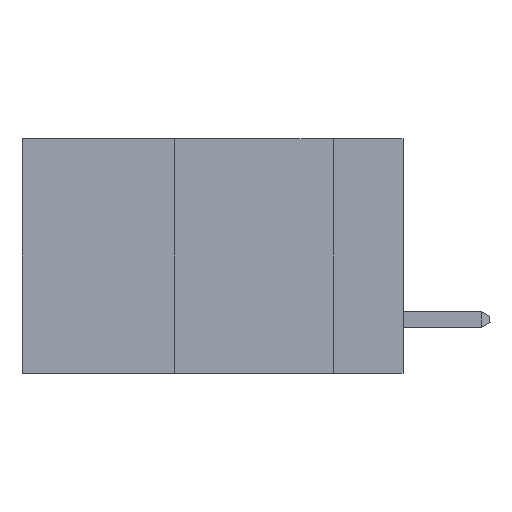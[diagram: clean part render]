
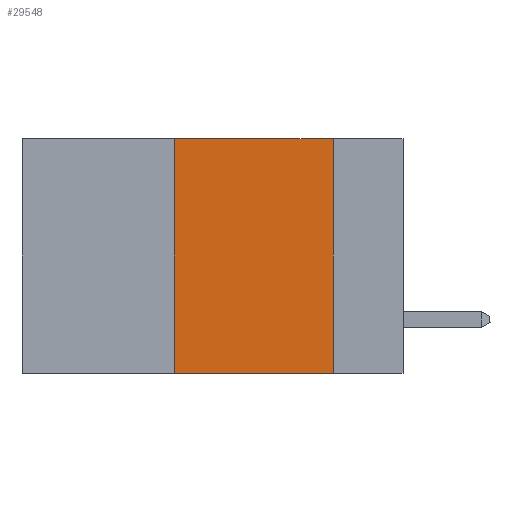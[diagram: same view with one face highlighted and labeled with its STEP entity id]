
A CAD part, left-side view. The second image highlights one B-rep face of the part: STEP entity #29548.
In plain terms, the highlighted planar face has unit normal (-1, 0, 0).
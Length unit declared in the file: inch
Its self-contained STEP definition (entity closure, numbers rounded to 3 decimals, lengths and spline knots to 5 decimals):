
#2512 = DIRECTION ( 'NONE',  ( 0., -1., 0. ) ) ;
#3248 = EDGE_CURVE ( 'NONE', #17567, #26143, #38191, .T. ) ;
#7248 = ORIENTED_EDGE ( 'NONE', *, *, #3248, .T. ) ;
#9143 = FACE_OUTER_BOUND ( 'NONE', #29233, .T. ) ;
#9183 = VECTOR ( 'NONE', #2512, 39.37008 ) ;
#13706 = VECTOR ( 'NONE', #22675, 39.37008 ) ;
#14139 = ORIENTED_EDGE ( 'NONE', *, *, #31482, .F. ) ;
#14521 = CARTESIAN_POINT ( 'NONE',  ( 0., 0.6, 0. ) ) ;
#14981 = LINE ( 'NONE', #34038, #13706 ) ;
#17039 = DIRECTION ( 'NONE',  ( 0., -1., 0. ) ) ;
#17567 = VERTEX_POINT ( 'NONE', #29278 ) ;
#18116 = LINE ( 'NONE', #24671, #36914 ) ;
#18705 = VERTEX_POINT ( 'NONE', #47653 ) ;
#19003 = LINE ( 'NONE', #14521, #9183 ) ;
#21620 = AXIS2_PLACEMENT_3D ( 'NONE', #41394, #22061, #49184 ) ;
#22061 = DIRECTION ( 'NONE',  ( 1., 0., 0. ) ) ;
#22595 = ORIENTED_EDGE ( 'NONE', *, *, #48093, .F. ) ;
#22675 = DIRECTION ( 'NONE',  ( 0., 0., 1. ) ) ;
#24671 = CARTESIAN_POINT ( 'NONE',  ( 0., 0.11, 0. ) ) ;
#26143 = VERTEX_POINT ( 'NONE', #26427 ) ;
#26427 = CARTESIAN_POINT ( 'NONE',  ( 0., 0.11, -0.37 ) ) ;
#27709 = DIRECTION ( 'NONE',  ( 0., 0., -1. ) ) ;
#29233 = EDGE_LOOP ( 'NONE', ( #14139, #22595, #47042, #7248 ) ) ;
#29278 = CARTESIAN_POINT ( 'NONE',  ( 0., 0.36, -0.37 ) ) ;
#29548 = ADVANCED_FACE ( 'NONE', ( #9143 ), #45267, .F. ) ;
#31482 = EDGE_CURVE ( 'NONE', #18705, #26143, #18116, .T. ) ;
#34038 = CARTESIAN_POINT ( 'NONE',  ( 0., 0.36, 0. ) ) ;
#34931 = CARTESIAN_POINT ( 'NONE',  ( 0., 0.36, 0. ) ) ;
#36106 = EDGE_CURVE ( 'NONE', #17567, #45476, #14981, .T. ) ;
#36914 = VECTOR ( 'NONE', #27709, 39.37008 ) ;
#38191 = LINE ( 'NONE', #40271, #44687 ) ;
#40271 = CARTESIAN_POINT ( 'NONE',  ( 0., 0.6, -0.37 ) ) ;
#41394 = CARTESIAN_POINT ( 'NONE',  ( 0., 0.6, 0. ) ) ;
#44687 = VECTOR ( 'NONE', #17039, 39.37008 ) ;
#45267 = PLANE ( 'NONE',  #21620 ) ;
#45476 = VERTEX_POINT ( 'NONE', #34931 ) ;
#47042 = ORIENTED_EDGE ( 'NONE', *, *, #36106, .F. ) ;
#47653 = CARTESIAN_POINT ( 'NONE',  ( 0., 0.11, 0. ) ) ;
#48093 = EDGE_CURVE ( 'NONE', #45476, #18705, #19003, .T. ) ;
#49184 = DIRECTION ( 'NONE',  ( 0., 0., -1. ) ) ;
